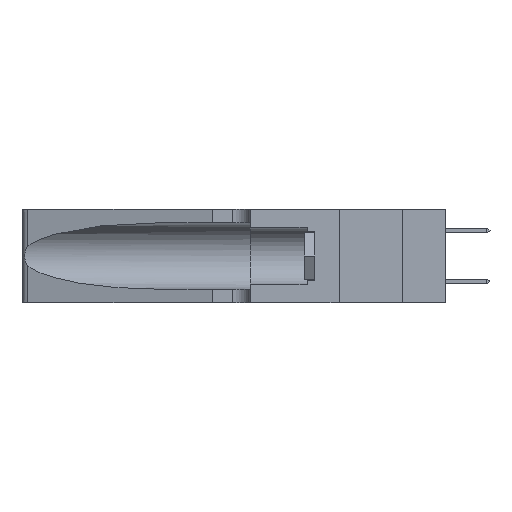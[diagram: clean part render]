
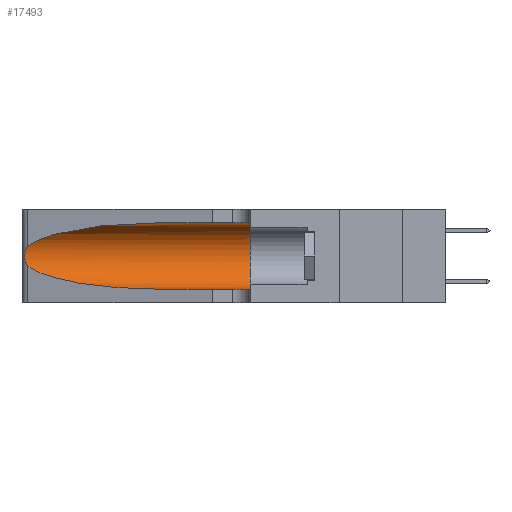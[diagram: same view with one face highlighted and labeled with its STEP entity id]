
A CAD part, left-side view. The second image highlights one B-rep face of the part: STEP entity #17493.
In plain terms, the highlighted cylindrical face has radius 3.308 mm (diameter 6.617 mm), a partial arc.
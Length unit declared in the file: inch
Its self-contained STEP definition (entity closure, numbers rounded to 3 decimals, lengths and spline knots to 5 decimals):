
#336 = EDGE_LOOP ( 'NONE', ( #16722, #16323, #14755, #17334, #21009, #2938 ) ) ;
#939 = DIRECTION ( 'NONE',  ( 0., 0., 1. ) ) ;
#997 = CARTESIAN_POINT ( 'NONE',  ( 0.25555, 1.22994, 0.2215 ) ) ;
#1092 = CARTESIAN_POINT ( 'NONE',  ( 0.26075, 1.23896, 0.19203 ) ) ;
#1117 = EDGE_CURVE ( 'NONE', #21090, #9909, #13411, .T. ) ;
#1691 = CARTESIAN_POINT ( 'NONE',  ( 0.18966, 0.96281, 0.31525 ) ) ;
#1877 = AXIS2_PLACEMENT_3D ( 'NONE', #6823, #18537, #6649 ) ;
#2086 = AXIS2_PLACEMENT_3D ( 'NONE', #10873, #20645, #939 ) ;
#2938 = ORIENTED_EDGE ( 'NONE', *, *, #13537, .F. ) ;
#3080 = CARTESIAN_POINT ( 'NONE',  ( 0.25555, 1.22993, 0.14849 ) ) ;
#3607 = LINE ( 'NONE', #22214, #4805 ) ;
#4040 = CARTESIAN_POINT ( 'NONE',  ( 0.25487, 1.22718, 0.14631 ) ) ;
#4357 = DIRECTION ( 'NONE',  ( 0., -1., 0. ) ) ;
#4711 = CARTESIAN_POINT ( 'NONE',  ( 0.18966, 0.96281, 0.05475 ) ) ;
#4805 = VECTOR ( 'NONE', #4357, 39.37008 ) ;
#5164 = CARTESIAN_POINT ( 'NONE',  ( 0.25487, 1.22718, 0.14631 ) ) ;
#5264 = CARTESIAN_POINT ( 'NONE',  ( 0.25487, 1.22718, 0.14631 ) ) ;
#5452 = EDGE_CURVE ( 'NONE', #17935, #23941, #9574, .T. ) ;
#6649 = DIRECTION ( 'NONE',  ( 0., 0., -1. ) ) ;
#6823 = CARTESIAN_POINT ( 'NONE',  ( 0.1305, 1.61858, 0.185 ) ) ;
#6914 = CARTESIAN_POINT ( 'NONE',  ( 0.26018, 1.23835, 0.19895 ) ) ;
#7526 = EDGE_CURVE ( 'NONE', #10562, #21090, #8107, .T. ) ;
#7536 = FACE_OUTER_BOUND ( 'NONE', #336, .T. ) ;
#8107 =( BOUNDED_CURVE ( )  B_SPLINE_CURVE ( 3, ( #4040, #23851, #4711, #20598 ),
 .UNSPECIFIED., .F., .T. ) 
 B_SPLINE_CURVE_WITH_KNOTS ( ( 4, 4 ),
 ( 3.44316, 4.71239 ),
 .UNSPECIFIED. ) 
 CURVE ( )  GEOMETRIC_REPRESENTATION_ITEM ( )  RATIONAL_B_SPLINE_CURVE ( ( 1., 0.87, 0.87, 1. ) ) 
 REPRESENTATION_ITEM ( '' )  );
#9139 = DIRECTION ( 'NONE',  ( 0., -1., 0. ) ) ;
#9242 = CARTESIAN_POINT ( 'NONE',  ( 0.26075, 1.23896, 0.178 ) ) ;
#9379 = CARTESIAN_POINT ( 'NONE',  ( 0.1305, 0.35, 0.05475 ) ) ;
#9574 =( BOUNDED_CURVE ( )  B_SPLINE_CURVE ( 3, ( #13617, #1691, #15598, #19753 ),
 .UNSPECIFIED., .F., .F. ) 
 B_SPLINE_CURVE_WITH_KNOTS ( ( 4, 4 ),
 ( 1.5708, 2.84003 ),
 .UNSPECIFIED. ) 
 CURVE ( )  GEOMETRIC_REPRESENTATION_ITEM ( )  RATIONAL_B_SPLINE_CURVE ( ( 1., 0.87, 0.87, 1. ) ) 
 REPRESENTATION_ITEM ( '' )  );
#9909 = VERTEX_POINT ( 'NONE', #9379 ) ;
#10283 = VECTOR ( 'NONE', #9139, 39.37008 ) ;
#10557 = CARTESIAN_POINT ( 'NONE',  ( 0.1305, 0.72297, 0.31525 ) ) ;
#10562 = VERTEX_POINT ( 'NONE', #5264 ) ;
#10873 = CARTESIAN_POINT ( 'NONE',  ( 0.1305, 0.35, 0.185 ) ) ;
#10916 = CARTESIAN_POINT ( 'NONE',  ( 0.1305, 1.61858, 0.05475 ) ) ;
#11099 = CARTESIAN_POINT ( 'NONE',  ( 0.25787, 1.23484, 0.2124 ) ) ;
#11350 = EDGE_CURVE ( 'NONE', #16272, #9909, #16149, .T. ) ;
#13007 = CARTESIAN_POINT ( 'NONE',  ( 0.26017, 1.23833, 0.17102 ) ) ;
#13090 = CARTESIAN_POINT ( 'NONE',  ( 0.25639, 1.23186, 0.15144 ) ) ;
#13411 = LINE ( 'NONE', #10916, #10283 ) ;
#13537 = EDGE_CURVE ( 'NONE', #17935, #16272, #3607, .T. ) ;
#13617 = CARTESIAN_POINT ( 'NONE',  ( 0.1305, 0.72297, 0.31525 ) ) ;
#14755 = ORIENTED_EDGE ( 'NONE', *, *, #7526, .T. ) ;
#14992 = CARTESIAN_POINT ( 'NONE',  ( 0.25789, 1.23486, 0.15765 ) ) ;
#15162 = CARTESIAN_POINT ( 'NONE',  ( 0.25856, 1.23593, 0.16098 ) ) ;
#15536 = EDGE_CURVE ( 'NONE', #23941, #10562, #24116, .T. ) ;
#15598 = CARTESIAN_POINT ( 'NONE',  ( 0.2373, 1.15595, 0.28018 ) ) ;
#16149 = CIRCLE ( 'NONE', #2086, 0.13025 ) ;
#16272 = VERTEX_POINT ( 'NONE', #19200 ) ;
#16323 = ORIENTED_EDGE ( 'NONE', *, *, #15536, .T. ) ;
#16722 = ORIENTED_EDGE ( 'NONE', *, *, #5452, .T. ) ;
#17334 = ORIENTED_EDGE ( 'NONE', *, *, #1117, .T. ) ;
#17493 = ADVANCED_FACE ( 'NONE', ( #7536 ), #21810, .F. ) ;
#17935 = VERTEX_POINT ( 'NONE', #10557 ) ;
#18537 = DIRECTION ( 'NONE',  ( 0., -1., 0. ) ) ;
#19041 = CARTESIAN_POINT ( 'NONE',  ( 0.25487, 1.22718, 0.22369 ) ) ;
#19200 = CARTESIAN_POINT ( 'NONE',  ( 0.1305, 0.35, 0.31525 ) ) ;
#19753 = CARTESIAN_POINT ( 'NONE',  ( 0.25487, 1.22718, 0.22369 ) ) ;
#20598 = CARTESIAN_POINT ( 'NONE',  ( 0.1305, 0.72297, 0.05475 ) ) ;
#20645 = DIRECTION ( 'NONE',  ( 0., 1., 0. ) ) ;
#20909 = CARTESIAN_POINT ( 'NONE',  ( 0.25487, 1.22718, 0.22369 ) ) ;
#21009 = ORIENTED_EDGE ( 'NONE', *, *, #11350, .F. ) ;
#21090 = VERTEX_POINT ( 'NONE', #25589 ) ;
#21810 = CYLINDRICAL_SURFACE ( 'NONE', #1877, 0.13025 ) ;
#22214 = CARTESIAN_POINT ( 'NONE',  ( 0.1305, 1.61858, 0.31525 ) ) ;
#22922 = CARTESIAN_POINT ( 'NONE',  ( 0.25639, 1.23184, 0.21858 ) ) ;
#23851 = CARTESIAN_POINT ( 'NONE',  ( 0.2373, 1.15595, 0.08982 ) ) ;
#23941 = VERTEX_POINT ( 'NONE', #20909 ) ;
#24116 = B_SPLINE_CURVE_WITH_KNOTS ( 'NONE', 3,
 ( #19041, #997, #22922, #11099, #24879, #6914, #1092, #9242, #13007, #15162, #14992, #13090, #3080, #5164 ),
 .UNSPECIFIED., .F., .F.,
 ( 4, 2, 2, 2, 2, 2, 4 ),
 ( 0., 0.00027, 0.00053, 0.00107, 0.0016, 0.00187, 0.00214 ),
 .UNSPECIFIED. ) ;
#24879 = CARTESIAN_POINT ( 'NONE',  ( 0.25854, 1.2359, 0.20912 ) ) ;
#25589 = CARTESIAN_POINT ( 'NONE',  ( 0.1305, 0.72297, 0.05475 ) ) ;
